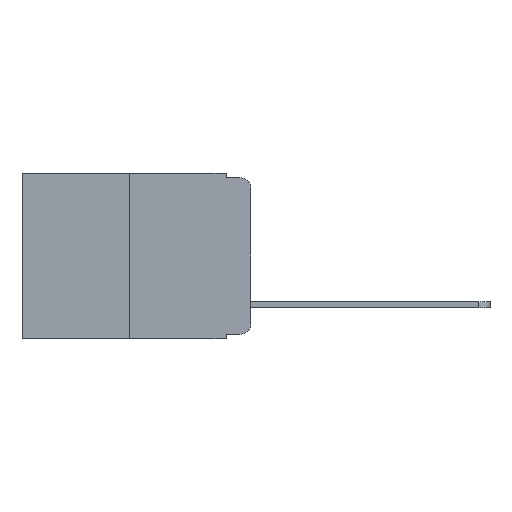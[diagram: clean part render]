
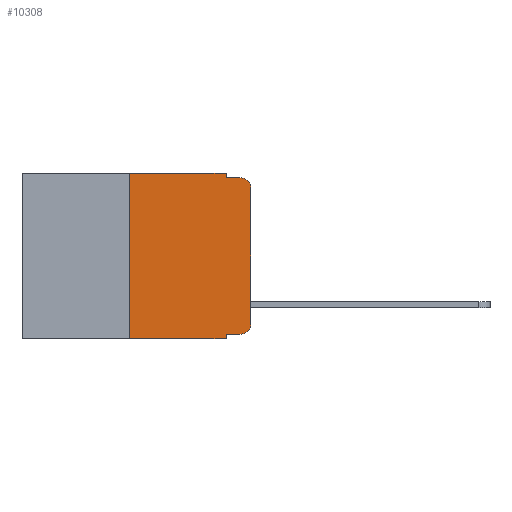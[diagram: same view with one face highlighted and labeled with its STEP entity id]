
A CAD part, left-side view. The second image highlights one B-rep face of the part: STEP entity #10308.
In plain terms, the highlighted planar face has unit normal (-1, 0, 0).
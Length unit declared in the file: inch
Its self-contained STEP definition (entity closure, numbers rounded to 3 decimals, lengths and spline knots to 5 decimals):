
#44 = LINE ( 'NONE', #2728, #1912 ) ;
#233 = VECTOR ( 'NONE', #5805, 39.37008 ) ;
#252 = AXIS2_PLACEMENT_3D ( 'NONE', #8096, #3856, #9799 ) ;
#380 = DIRECTION ( 'NONE',  ( 0., 0., -1. ) ) ;
#558 = ORIENTED_EDGE ( 'NONE', *, *, #7241, .T. ) ;
#600 = CARTESIAN_POINT ( 'NONE',  ( 0., 0.051, -0.343 ) ) ;
#640 = FACE_OUTER_BOUND ( 'NONE', #7207, .T. ) ;
#641 = DIRECTION ( 'NONE',  ( -1., 0., 0. ) ) ;
#777 = VERTEX_POINT ( 'NONE', #2297 ) ;
#1077 = CIRCLE ( 'NONE', #7925, 0.02 ) ;
#1134 = DIRECTION ( 'NONE',  ( 0., 0., 1. ) ) ;
#1285 = CARTESIAN_POINT ( 'NONE',  ( 0., 0.051, -0.333 ) ) ;
#1434 = LINE ( 'NONE', #9445, #9941 ) ;
#1715 = VERTEX_POINT ( 'NONE', #2839 ) ;
#1912 = VECTOR ( 'NONE', #1134, 39.37008 ) ;
#2145 = DIRECTION ( 'NONE',  ( 0., -1., 0. ) ) ;
#2162 = ORIENTED_EDGE ( 'NONE', *, *, #6882, .T. ) ;
#2297 = CARTESIAN_POINT ( 'NONE',  ( 0., 0.25, 0. ) ) ;
#2345 = CARTESIAN_POINT ( 'NONE',  ( 0., 0.02, -0.313 ) ) ;
#2382 = LINE ( 'NONE', #1285, #6626 ) ;
#2386 = CARTESIAN_POINT ( 'NONE',  ( 0., 0.473, -0.343 ) ) ;
#2425 = EDGE_CURVE ( 'NONE', #5570, #777, #44, .T. ) ;
#2492 = LINE ( 'NONE', #4053, #233 ) ;
#2728 = CARTESIAN_POINT ( 'NONE',  ( 0., 0.25, 0. ) ) ;
#2839 = CARTESIAN_POINT ( 'NONE',  ( 0., 0., -0.03 ) ) ;
#2918 = VECTOR ( 'NONE', #6565, 39.37008 ) ;
#3142 = EDGE_CURVE ( 'NONE', #3618, #6892, #8157, .T. ) ;
#3249 = LINE ( 'NONE', #3661, #7088 ) ;
#3394 = DIRECTION ( 'NONE',  ( 0., 0., 1. ) ) ;
#3421 = DIRECTION ( 'NONE',  ( 0., 0., -1. ) ) ;
#3618 = VERTEX_POINT ( 'NONE', #7873 ) ;
#3661 = CARTESIAN_POINT ( 'NONE',  ( 0., 0.473, 0. ) ) ;
#3856 = DIRECTION ( 'NONE',  ( 1., 0., 0. ) ) ;
#3886 = EDGE_CURVE ( 'NONE', #777, #7263, #3249, .T. ) ;
#4053 = CARTESIAN_POINT ( 'NONE',  ( 0., 0.051, -0.01 ) ) ;
#4593 = VECTOR ( 'NONE', #3421, 39.37008 ) ;
#4603 = DIRECTION ( 'NONE',  ( 0., 0., -1. ) ) ;
#4659 = CIRCLE ( 'NONE', #10709, 0.02 ) ;
#4709 = CARTESIAN_POINT ( 'NONE',  ( 0., 0.051, 0. ) ) ;
#4836 = EDGE_CURVE ( 'NONE', #5570, #6892, #5165, .T. ) ;
#5165 = LINE ( 'NONE', #2386, #2918 ) ;
#5207 = VERTEX_POINT ( 'NONE', #7670 ) ;
#5281 = ORIENTED_EDGE ( 'NONE', *, *, #10569, .T. ) ;
#5289 = ORIENTED_EDGE ( 'NONE', *, *, #3886, .F. ) ;
#5353 = CARTESIAN_POINT ( 'NONE',  ( 0., 0.02, -0.03 ) ) ;
#5372 = DIRECTION ( 'NONE',  ( 0., -1., 0. ) ) ;
#5570 = VERTEX_POINT ( 'NONE', #6607 ) ;
#5743 = VERTEX_POINT ( 'NONE', #5897 ) ;
#5805 = DIRECTION ( 'NONE',  ( 0., -1., 0. ) ) ;
#5885 = CARTESIAN_POINT ( 'NONE',  ( 0., 0., -0.313 ) ) ;
#5887 = VECTOR ( 'NONE', #380, 39.37008 ) ;
#5897 = CARTESIAN_POINT ( 'NONE',  ( 0., 0.051, -0.01 ) ) ;
#6217 = ORIENTED_EDGE ( 'NONE', *, *, #8358, .F. ) ;
#6403 = VERTEX_POINT ( 'NONE', #5885 ) ;
#6565 = DIRECTION ( 'NONE',  ( 0., -1., 0. ) ) ;
#6607 = CARTESIAN_POINT ( 'NONE',  ( 0., 0.25, -0.343 ) ) ;
#6626 = VECTOR ( 'NONE', #2145, 39.37008 ) ;
#6756 = ORIENTED_EDGE ( 'NONE', *, *, #4836, .T. ) ;
#6882 = EDGE_CURVE ( 'NONE', #5207, #6403, #1077, .T. ) ;
#6892 = VERTEX_POINT ( 'NONE', #600 ) ;
#7088 = VECTOR ( 'NONE', #5372, 39.37008 ) ;
#7207 = EDGE_LOOP ( 'NONE', ( #5281, #558, #6217, #9258, #5289, #8391, #6756, #9309, #7723, #2162 ) ) ;
#7241 = EDGE_CURVE ( 'NONE', #1715, #10018, #4659, .T. ) ;
#7263 = VERTEX_POINT ( 'NONE', #10538 ) ;
#7344 = PLANE ( 'NONE',  #252 ) ;
#7392 = LINE ( 'NONE', #7548, #4593 ) ;
#7548 = CARTESIAN_POINT ( 'NONE',  ( 0., 0.051, 0. ) ) ;
#7670 = CARTESIAN_POINT ( 'NONE',  ( 0., 0.02, -0.333 ) ) ;
#7723 = ORIENTED_EDGE ( 'NONE', *, *, #10293, .T. ) ;
#7873 = CARTESIAN_POINT ( 'NONE',  ( 0., 0.051, -0.333 ) ) ;
#7925 = AXIS2_PLACEMENT_3D ( 'NONE', #2345, #641, #9989 ) ;
#8096 = CARTESIAN_POINT ( 'NONE',  ( 0., 0.473, 0. ) ) ;
#8157 = LINE ( 'NONE', #4709, #5887 ) ;
#8358 = EDGE_CURVE ( 'NONE', #5743, #10018, #2492, .T. ) ;
#8391 = ORIENTED_EDGE ( 'NONE', *, *, #2425, .F. ) ;
#9009 = EDGE_CURVE ( 'NONE', #7263, #5743, #7392, .T. ) ;
#9258 = ORIENTED_EDGE ( 'NONE', *, *, #9009, .F. ) ;
#9309 = ORIENTED_EDGE ( 'NONE', *, *, #3142, .F. ) ;
#9445 = CARTESIAN_POINT ( 'NONE',  ( 0., 0., 0. ) ) ;
#9545 = DIRECTION ( 'NONE',  ( -1., 0., 0. ) ) ;
#9799 = DIRECTION ( 'NONE',  ( 0., 0., -1. ) ) ;
#9941 = VECTOR ( 'NONE', #3394, 39.37008 ) ;
#9989 = DIRECTION ( 'NONE',  ( 0., 0., -1. ) ) ;
#10018 = VERTEX_POINT ( 'NONE', #10400 ) ;
#10293 = EDGE_CURVE ( 'NONE', #3618, #5207, #2382, .T. ) ;
#10308 = ADVANCED_FACE ( 'NONE', ( #640 ), #7344, .F. ) ;
#10400 = CARTESIAN_POINT ( 'NONE',  ( 0., 0.02, -0.01 ) ) ;
#10538 = CARTESIAN_POINT ( 'NONE',  ( 0., 0.051, 0. ) ) ;
#10569 = EDGE_CURVE ( 'NONE', #6403, #1715, #1434, .T. ) ;
#10709 = AXIS2_PLACEMENT_3D ( 'NONE', #5353, #9545, #4603 ) ;
